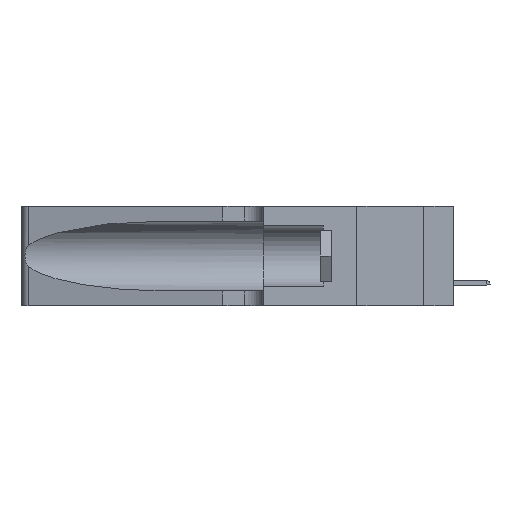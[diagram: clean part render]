
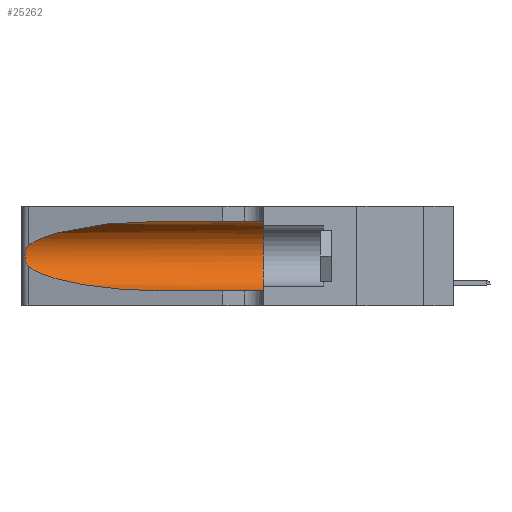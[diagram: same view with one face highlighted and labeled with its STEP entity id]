
A CAD part, left-side view. The second image highlights one B-rep face of the part: STEP entity #25262.
In plain terms, the highlighted cylindrical face has radius 3.308 mm (diameter 6.617 mm), a partial arc.
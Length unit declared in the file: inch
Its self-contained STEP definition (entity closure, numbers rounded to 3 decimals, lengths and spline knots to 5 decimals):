
#898 = CARTESIAN_POINT ( 'NONE',  ( 0.1305, 0.35, 0.185 ) ) ;
#1281 = ORIENTED_EDGE ( 'NONE', *, *, #9939, .F. ) ;
#1370 = CARTESIAN_POINT ( 'NONE',  ( 0.25787, 1.23484, 0.2124 ) ) ;
#1657 = CARTESIAN_POINT ( 'NONE',  ( 0.26017, 1.23833, 0.17102 ) ) ;
#1803 = CARTESIAN_POINT ( 'NONE',  ( 0.25639, 1.23184, 0.21858 ) ) ;
#3091 = VERTEX_POINT ( 'NONE', #25557 ) ;
#3540 = CARTESIAN_POINT ( 'NONE',  ( 0.26075, 1.23896, 0.19203 ) ) ;
#3750 = AXIS2_PLACEMENT_3D ( 'NONE', #898, #27202, #25170 ) ;
#3837 = CARTESIAN_POINT ( 'NONE',  ( 0.25789, 1.23486, 0.15765 ) ) ;
#3979 = CARTESIAN_POINT ( 'NONE',  ( 0.25555, 1.22994, 0.2215 ) ) ;
#5163 = ORIENTED_EDGE ( 'NONE', *, *, #26879, .T. ) ;
#5654 = CARTESIAN_POINT ( 'NONE',  ( 0.18966, 0.96281, 0.31525 ) ) ;
#6117 = VERTEX_POINT ( 'NONE', #13611 ) ;
#6265 = DIRECTION ( 'NONE',  ( 0., -1., 0. ) ) ;
#6473 = B_SPLINE_CURVE_WITH_KNOTS ( 'NONE', 3,
 ( #21361, #3979, #1803, #1370, #12459, #10166, #3540, #10440, #1657, #19340, #3837, #14736, #23521, #23795 ),
 .UNSPECIFIED., .F., .F.,
 ( 4, 2, 2, 2, 2, 2, 4 ),
 ( 0., 0.00027, 0.00053, 0.00107, 0.0016, 0.00187, 0.00214 ),
 .UNSPECIFIED. ) ;
#7143 = DIRECTION ( 'NONE',  ( 0., -1., 0. ) ) ;
#7939 = CARTESIAN_POINT ( 'NONE',  ( 0.25487, 1.22718, 0.22369 ) ) ;
#8580 = EDGE_CURVE ( 'NONE', #12251, #3091, #10674, .T. ) ;
#8736 = CARTESIAN_POINT ( 'NONE',  ( 0.1305, 0.35, 0.31525 ) ) ;
#9055 = VERTEX_POINT ( 'NONE', #27871 ) ;
#9614 = EDGE_CURVE ( 'NONE', #26930, #6117, #16018, .T. ) ;
#9939 = EDGE_CURVE ( 'NONE', #26930, #21932, #10860, .T. ) ;
#10166 = CARTESIAN_POINT ( 'NONE',  ( 0.26018, 1.23835, 0.19895 ) ) ;
#10440 = CARTESIAN_POINT ( 'NONE',  ( 0.26075, 1.23896, 0.178 ) ) ;
#10674 = LINE ( 'NONE', #19279, #27079 ) ;
#10860 = LINE ( 'NONE', #17173, #23485 ) ;
#11737 = CYLINDRICAL_SURFACE ( 'NONE', #18935, 0.13025 ) ;
#12251 = VERTEX_POINT ( 'NONE', #14215 ) ;
#12459 = CARTESIAN_POINT ( 'NONE',  ( 0.25854, 1.2359, 0.20912 ) ) ;
#12531 = CARTESIAN_POINT ( 'NONE',  ( 0.1305, 0.72297, 0.31525 ) ) ;
#13258 = CARTESIAN_POINT ( 'NONE',  ( 0.1305, 0.72297, 0.05475 ) ) ;
#13611 = CARTESIAN_POINT ( 'NONE',  ( 0.25487, 1.22718, 0.22369 ) ) ;
#14215 = CARTESIAN_POINT ( 'NONE',  ( 0.1305, 0.72297, 0.05475 ) ) ;
#14736 = CARTESIAN_POINT ( 'NONE',  ( 0.25639, 1.23186, 0.15144 ) ) ;
#15403 = CARTESIAN_POINT ( 'NONE',  ( 0.18966, 0.96281, 0.05475 ) ) ;
#15894 = DIRECTION ( 'NONE',  ( 0., 0., -1. ) ) ;
#16018 =( BOUNDED_CURVE ( )  B_SPLINE_CURVE ( 3, ( #12531, #5654, #27613, #7939 ),
 .UNSPECIFIED., .F., .T. ) 
 B_SPLINE_CURVE_WITH_KNOTS ( ( 4, 4 ),
 ( 1.5708, 2.84003 ),
 .UNSPECIFIED. ) 
 CURVE ( )  GEOMETRIC_REPRESENTATION_ITEM ( )  RATIONAL_B_SPLINE_CURVE ( ( 1., 0.87, 0.87, 1. ) ) 
 REPRESENTATION_ITEM ( '' )  );
#17173 = CARTESIAN_POINT ( 'NONE',  ( 0.1305, 1.61858, 0.31525 ) ) ;
#17240 = ORIENTED_EDGE ( 'NONE', *, *, #8580, .T. ) ;
#18935 = AXIS2_PLACEMENT_3D ( 'NONE', #22510, #7143, #15894 ) ;
#18965 =( BOUNDED_CURVE ( )  B_SPLINE_CURVE ( 3, ( #22302, #24302, #15403, #13258 ),
 .UNSPECIFIED., .F., .T. ) 
 B_SPLINE_CURVE_WITH_KNOTS ( ( 4, 4 ),
 ( 3.44316, 4.71239 ),
 .UNSPECIFIED. ) 
 CURVE ( )  GEOMETRIC_REPRESENTATION_ITEM ( )  RATIONAL_B_SPLINE_CURVE ( ( 1., 0.87, 0.87, 1. ) ) 
 REPRESENTATION_ITEM ( '' )  );
#19279 = CARTESIAN_POINT ( 'NONE',  ( 0.1305, 1.61858, 0.05475 ) ) ;
#19340 = CARTESIAN_POINT ( 'NONE',  ( 0.25856, 1.23593, 0.16098 ) ) ;
#19416 = DIRECTION ( 'NONE',  ( 0., -1., 0. ) ) ;
#20257 = CIRCLE ( 'NONE', #3750, 0.13025 ) ;
#20561 = ORIENTED_EDGE ( 'NONE', *, *, #9614, .T. ) ;
#21361 = CARTESIAN_POINT ( 'NONE',  ( 0.25487, 1.22718, 0.22369 ) ) ;
#21808 = ORIENTED_EDGE ( 'NONE', *, *, #23840, .F. ) ;
#21932 = VERTEX_POINT ( 'NONE', #8736 ) ;
#22302 = CARTESIAN_POINT ( 'NONE',  ( 0.25487, 1.22718, 0.14631 ) ) ;
#22510 = CARTESIAN_POINT ( 'NONE',  ( 0.1305, 1.61858, 0.185 ) ) ;
#22789 = FACE_OUTER_BOUND ( 'NONE', #25039, .T. ) ;
#23485 = VECTOR ( 'NONE', #6265, 39.37008 ) ;
#23521 = CARTESIAN_POINT ( 'NONE',  ( 0.25555, 1.22993, 0.14849 ) ) ;
#23795 = CARTESIAN_POINT ( 'NONE',  ( 0.25487, 1.22718, 0.14631 ) ) ;
#23840 = EDGE_CURVE ( 'NONE', #21932, #3091, #20257, .T. ) ;
#24302 = CARTESIAN_POINT ( 'NONE',  ( 0.2373, 1.15595, 0.08982 ) ) ;
#25039 = EDGE_LOOP ( 'NONE', ( #20561, #27985, #5163, #17240, #21808, #1281 ) ) ;
#25170 = DIRECTION ( 'NONE',  ( 0., 0., 1. ) ) ;
#25262 = ADVANCED_FACE ( 'NONE', ( #22789 ), #11737, .F. ) ;
#25557 = CARTESIAN_POINT ( 'NONE',  ( 0.1305, 0.35, 0.05475 ) ) ;
#26299 = EDGE_CURVE ( 'NONE', #6117, #9055, #6473, .T. ) ;
#26759 = CARTESIAN_POINT ( 'NONE',  ( 0.1305, 0.72297, 0.31525 ) ) ;
#26879 = EDGE_CURVE ( 'NONE', #9055, #12251, #18965, .T. ) ;
#26930 = VERTEX_POINT ( 'NONE', #26759 ) ;
#27079 = VECTOR ( 'NONE', #19416, 39.37008 ) ;
#27202 = DIRECTION ( 'NONE',  ( 0., 1., 0. ) ) ;
#27613 = CARTESIAN_POINT ( 'NONE',  ( 0.2373, 1.15595, 0.28018 ) ) ;
#27871 = CARTESIAN_POINT ( 'NONE',  ( 0.25487, 1.22718, 0.14631 ) ) ;
#27985 = ORIENTED_EDGE ( 'NONE', *, *, #26299, .T. ) ;
